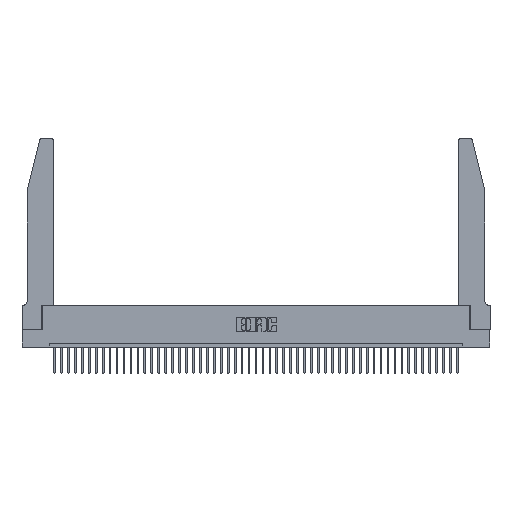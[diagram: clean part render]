
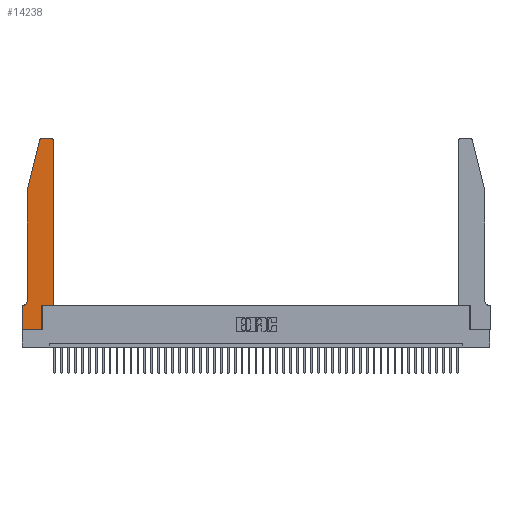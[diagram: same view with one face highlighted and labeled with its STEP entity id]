
A CAD part, top view. The second image highlights one B-rep face of the part: STEP entity #14238.
In plain terms, the highlighted planar face has unit normal (0, 0, 1).
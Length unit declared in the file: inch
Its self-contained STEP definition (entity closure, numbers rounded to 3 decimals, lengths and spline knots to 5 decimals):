
#637 = ORIENTED_EDGE ( 'NONE', *, *, #33693, .T. ) ;
#779 = VECTOR ( 'NONE', #16818, 39.37008 ) ;
#783 = ORIENTED_EDGE ( 'NONE', *, *, #8712, .T. ) ;
#1207 = CARTESIAN_POINT ( 'NONE',  ( 0.284, 2.72, 0.37 ) ) ;
#1312 = EDGE_CURVE ( 'NONE', #27906, #21381, #18878, .T. ) ;
#1490 = DIRECTION ( 'NONE',  ( 1., 0., 0. ) ) ;
#1772 = LINE ( 'NONE', #17788, #40381 ) ;
#2111 = EDGE_LOOP ( 'NONE', ( #36159, #24840, #637, #11387, #21033, #11614, #17726, #11789, #783, #9489, #5297, #12270 ) ) ;
#2704 = CARTESIAN_POINT ( 'NONE',  ( 0.2865, 0., 0.37 ) ) ;
#2771 = LINE ( 'NONE', #7217, #8444 ) ;
#4551 = EDGE_CURVE ( 'NONE', #6547, #27906, #22223, .T. ) ;
#4662 = FACE_OUTER_BOUND ( 'NONE', #2111, .T. ) ;
#4682 = CARTESIAN_POINT ( 'NONE',  ( 0.284, 2.75, 0.37 ) ) ;
#4723 = EDGE_CURVE ( 'NONE', #21381, #6180, #1772, .T. ) ;
#5123 = DIRECTION ( 'NONE',  ( -1., 0., 0. ) ) ;
#5297 = ORIENTED_EDGE ( 'NONE', *, *, #46668, .T. ) ;
#5505 = CIRCLE ( 'NONE', #31910, 0.03 ) ;
#6180 = VERTEX_POINT ( 'NONE', #17499 ) ;
#6547 = VERTEX_POINT ( 'NONE', #34978 ) ;
#6872 = CARTESIAN_POINT ( 'NONE',  ( 0.4505, 0.35, 0.37 ) ) ;
#7217 = CARTESIAN_POINT ( 'NONE',  ( 0.0755, 2., 0.37 ) ) ;
#8062 = DIRECTION ( 'NONE',  ( 0., 0., 1. ) ) ;
#8444 = VECTOR ( 'NONE', #25285, 39.37008 ) ;
#8712 = EDGE_CURVE ( 'NONE', #12935, #27807, #45686, .T. ) ;
#9489 = ORIENTED_EDGE ( 'NONE', *, *, #9717, .T. ) ;
#9651 = VECTOR ( 'NONE', #20911, 39.37008 ) ;
#9717 = EDGE_CURVE ( 'NONE', #27807, #41159, #29683, .T. ) ;
#9910 = VECTOR ( 'NONE', #5123, 39.37008 ) ;
#11387 = ORIENTED_EDGE ( 'NONE', *, *, #38717, .T. ) ;
#11414 = LINE ( 'NONE', #45300, #25001 ) ;
#11509 = DIRECTION ( 'NONE',  ( -1., 0., 0. ) ) ;
#11614 = ORIENTED_EDGE ( 'NONE', *, *, #1312, .T. ) ;
#11789 = ORIENTED_EDGE ( 'NONE', *, *, #33168, .T. ) ;
#12118 = EDGE_CURVE ( 'NONE', #20328, #28982, #33271, .T. ) ;
#12270 = ORIENTED_EDGE ( 'NONE', *, *, #39563, .T. ) ;
#12935 = VERTEX_POINT ( 'NONE', #2704 ) ;
#13624 = DIRECTION ( 'NONE',  ( 1., 0., 0. ) ) ;
#13687 = EDGE_CURVE ( 'NONE', #28982, #38488, #23488, .T. ) ;
#14238 = ADVANCED_FACE ( 'NONE', ( #4662 ), #15513, .T. ) ;
#15513 = PLANE ( 'NONE',  #21840 ) ;
#16764 = CARTESIAN_POINT ( 'NONE',  ( 0.0755, 2., 0.37 ) ) ;
#16818 = DIRECTION ( 'NONE',  ( 0., 1., 0. ) ) ;
#17143 = CARTESIAN_POINT ( 'NONE',  ( 0.4505, 2.72, 0.37 ) ) ;
#17499 = CARTESIAN_POINT ( 'NONE',  ( 0., 0., 0.37 ) ) ;
#17535 = DIRECTION ( 'NONE',  ( 0., 0., 1. ) ) ;
#17726 = ORIENTED_EDGE ( 'NONE', *, *, #4723, .T. ) ;
#17788 = CARTESIAN_POINT ( 'NONE',  ( 0., 0., 0.37 ) ) ;
#18878 = LINE ( 'NONE', #19704, #9910 ) ;
#19213 = AXIS2_PLACEMENT_3D ( 'NONE', #32811, #32959, #11509 ) ;
#19704 = CARTESIAN_POINT ( 'NONE',  ( 0.0755, 0.35, 0.37 ) ) ;
#20127 = VECTOR ( 'NONE', #1490, 39.37008 ) ;
#20212 = VECTOR ( 'NONE', #39537, 39.37008 ) ;
#20328 = VERTEX_POINT ( 'NONE', #26993 ) ;
#20911 = DIRECTION ( 'NONE',  ( -0.239, -0.971, 0. ) ) ;
#21033 = ORIENTED_EDGE ( 'NONE', *, *, #4551, .T. ) ;
#21152 = CARTESIAN_POINT ( 'NONE',  ( 0.2865, 0.35, 0.37 ) ) ;
#21381 = VERTEX_POINT ( 'NONE', #36798 ) ;
#21840 = AXIS2_PLACEMENT_3D ( 'NONE', #31621, #17535, #13624 ) ;
#22223 = CIRCLE ( 'NONE', #19213, 0.07 ) ;
#22925 = DIRECTION ( 'NONE',  ( 1., 0., 0. ) ) ;
#22927 = DIRECTION ( 'NONE',  ( 1., 0., 0. ) ) ;
#23488 = CIRCLE ( 'NONE', #39439, 0.03 ) ;
#23518 = CARTESIAN_POINT ( 'NONE',  ( 0.25487, 2.72718, 0.37 ) ) ;
#23621 = DIRECTION ( 'NONE',  ( 1., 0., 0. ) ) ;
#24840 = ORIENTED_EDGE ( 'NONE', *, *, #13687, .T. ) ;
#25001 = VECTOR ( 'NONE', #23621, 39.37008 ) ;
#25080 = CARTESIAN_POINT ( 'NONE',  ( 0.0755, 2., 0.37 ) ) ;
#25285 = DIRECTION ( 'NONE',  ( 0., -1., 0. ) ) ;
#25297 = LINE ( 'NONE', #34880, #779 ) ;
#26400 = CARTESIAN_POINT ( 'NONE',  ( 0.0055, 0.35, 0.37 ) ) ;
#26880 = CARTESIAN_POINT ( 'NONE',  ( 0.4505, 0.35, 0.37 ) ) ;
#26993 = CARTESIAN_POINT ( 'NONE',  ( 0.4205, 2.75, 0.37 ) ) ;
#27807 = VERTEX_POINT ( 'NONE', #44660 ) ;
#27906 = VERTEX_POINT ( 'NONE', #26400 ) ;
#28365 = VERTEX_POINT ( 'NONE', #25080 ) ;
#28982 = VERTEX_POINT ( 'NONE', #4682 ) ;
#29120 = DIRECTION ( 'NONE',  ( -1., 0., 0. ) ) ;
#29683 = LINE ( 'NONE', #26880, #20127 ) ;
#29716 = CARTESIAN_POINT ( 'NONE',  ( 0.4205, 2.72, 0.37 ) ) ;
#30251 = DIRECTION ( 'NONE',  ( 0., 0., 1. ) ) ;
#30845 = CARTESIAN_POINT ( 'NONE',  ( 0.2605, 2.75, 0.37 ) ) ;
#30975 = VERTEX_POINT ( 'NONE', #17143 ) ;
#31621 = CARTESIAN_POINT ( 'NONE',  ( 0., 0.35, 0.37 ) ) ;
#31910 = AXIS2_PLACEMENT_3D ( 'NONE', #29716, #8062, #22925 ) ;
#32811 = CARTESIAN_POINT ( 'NONE',  ( 0.0055, 0.42, 0.37 ) ) ;
#32959 = DIRECTION ( 'NONE',  ( 0., 0., -1. ) ) ;
#33168 = EDGE_CURVE ( 'NONE', #6180, #12935, #11414, .T. ) ;
#33271 = LINE ( 'NONE', #30845, #40655 ) ;
#33693 = EDGE_CURVE ( 'NONE', #38488, #28365, #45857, .T. ) ;
#34880 = CARTESIAN_POINT ( 'NONE',  ( 0.4505, 0.35, 0.37 ) ) ;
#34978 = CARTESIAN_POINT ( 'NONE',  ( 0.0755, 0.42, 0.37 ) ) ;
#36159 = ORIENTED_EDGE ( 'NONE', *, *, #12118, .T. ) ;
#36798 = CARTESIAN_POINT ( 'NONE',  ( 0., 0.35, 0.37 ) ) ;
#38488 = VERTEX_POINT ( 'NONE', #23518 ) ;
#38717 = EDGE_CURVE ( 'NONE', #28365, #6547, #2771, .T. ) ;
#39439 = AXIS2_PLACEMENT_3D ( 'NONE', #1207, #30251, #22927 ) ;
#39537 = DIRECTION ( 'NONE',  ( 0., 1., 0. ) ) ;
#39563 = EDGE_CURVE ( 'NONE', #30975, #20328, #5505, .T. ) ;
#40381 = VECTOR ( 'NONE', #40754, 39.37008 ) ;
#40655 = VECTOR ( 'NONE', #29120, 39.37008 ) ;
#40754 = DIRECTION ( 'NONE',  ( 0., -1., 0. ) ) ;
#41159 = VERTEX_POINT ( 'NONE', #6872 ) ;
#44660 = CARTESIAN_POINT ( 'NONE',  ( 0.2865, 0.35, 0.37 ) ) ;
#45300 = CARTESIAN_POINT ( 'NONE',  ( 0., 0., 0.37 ) ) ;
#45686 = LINE ( 'NONE', #21152, #20212 ) ;
#45857 = LINE ( 'NONE', #16764, #9651 ) ;
#46668 = EDGE_CURVE ( 'NONE', #41159, #30975, #25297, .T. ) ;
